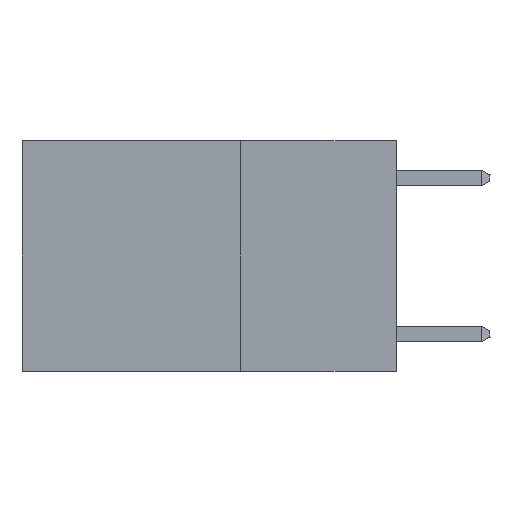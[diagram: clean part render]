
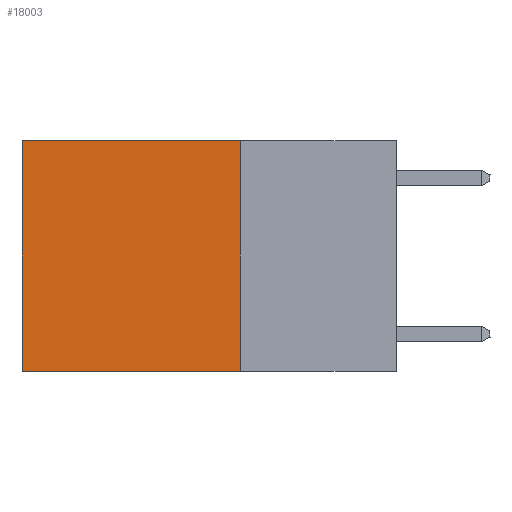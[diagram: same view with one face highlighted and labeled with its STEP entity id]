
A CAD part, left-side view. The second image highlights one B-rep face of the part: STEP entity #18003.
In plain terms, the highlighted planar face has unit normal (-1, 0, 0).
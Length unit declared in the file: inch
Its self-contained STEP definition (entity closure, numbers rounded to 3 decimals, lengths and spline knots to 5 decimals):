
#66 = VERTEX_POINT ( 'NONE', #347 ) ;
#262 = ORIENTED_EDGE ( 'NONE', *, *, #9144, .T. ) ;
#347 = CARTESIAN_POINT ( 'NONE',  ( 0.2625, 0.6, 0. ) ) ;
#698 = LINE ( 'NONE', #2215, #1901 ) ;
#1413 = DIRECTION ( 'NONE',  ( 0., 0., -1. ) ) ;
#1901 = VECTOR ( 'NONE', #7036, 39.37008 ) ;
#2015 = DIRECTION ( 'NONE',  ( 0., 1., 0. ) ) ;
#2215 = CARTESIAN_POINT ( 'NONE',  ( 0.2625, 0.25, 0. ) ) ;
#2226 = DIRECTION ( 'NONE',  ( 0., 0., -1. ) ) ;
#2320 = CARTESIAN_POINT ( 'NONE',  ( 0.2625, 0.6, -0.37 ) ) ;
#3081 = CARTESIAN_POINT ( 'NONE',  ( 0.2625, 0.6, 0. ) ) ;
#3375 = CARTESIAN_POINT ( 'NONE',  ( 0.2625, 0.25, 0. ) ) ;
#3912 = CARTESIAN_POINT ( 'NONE',  ( 0.2625, 0.25, 0. ) ) ;
#6208 = ORIENTED_EDGE ( 'NONE', *, *, #19592, .T. ) ;
#6220 = FACE_OUTER_BOUND ( 'NONE', #12735, .T. ) ;
#6766 = ORIENTED_EDGE ( 'NONE', *, *, #7152, .F. ) ;
#7036 = DIRECTION ( 'NONE',  ( 0., 1., 0. ) ) ;
#7152 = EDGE_CURVE ( 'NONE', #16346, #16990, #11711, .T. ) ;
#7588 = DIRECTION ( 'NONE',  ( 0., 0., -1. ) ) ;
#8411 = VECTOR ( 'NONE', #7588, 39.37008 ) ;
#9144 = EDGE_CURVE ( 'NONE', #17310, #66, #698, .T. ) ;
#9163 = CARTESIAN_POINT ( 'NONE',  ( 0.2625, 0.25, -0.37 ) ) ;
#10196 = VECTOR ( 'NONE', #2015, 39.37008 ) ;
#10757 = CARTESIAN_POINT ( 'NONE',  ( 0.2625, 0.25, 0. ) ) ;
#10996 = VECTOR ( 'NONE', #2226, 39.37008 ) ;
#11711 = LINE ( 'NONE', #15128, #10196 ) ;
#12487 = PLANE ( 'NONE',  #18267 ) ;
#12581 = EDGE_CURVE ( 'NONE', #17310, #16346, #16893, .T. ) ;
#12735 = EDGE_LOOP ( 'NONE', ( #6208, #6766, #15228, #262 ) ) ;
#15128 = CARTESIAN_POINT ( 'NONE',  ( 0.2625, 0.25, -0.37 ) ) ;
#15228 = ORIENTED_EDGE ( 'NONE', *, *, #12581, .F. ) ;
#16099 = DIRECTION ( 'NONE',  ( 1., 0., 0. ) ) ;
#16346 = VERTEX_POINT ( 'NONE', #9163 ) ;
#16893 = LINE ( 'NONE', #3912, #10996 ) ;
#16990 = VERTEX_POINT ( 'NONE', #2320 ) ;
#17310 = VERTEX_POINT ( 'NONE', #3375 ) ;
#18003 = ADVANCED_FACE ( 'NONE', ( #6220 ), #12487, .F. ) ;
#18267 = AXIS2_PLACEMENT_3D ( 'NONE', #10757, #16099, #1413 ) ;
#19592 = EDGE_CURVE ( 'NONE', #66, #16990, #20969, .T. ) ;
#20969 = LINE ( 'NONE', #3081, #8411 ) ;
